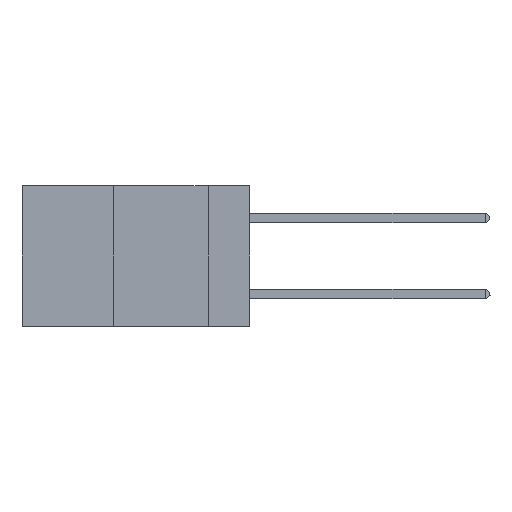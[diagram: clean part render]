
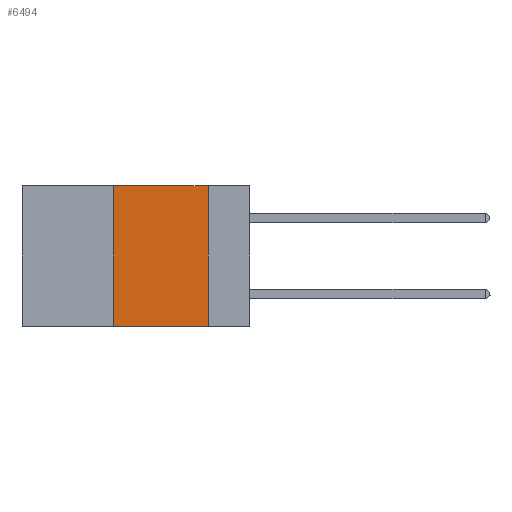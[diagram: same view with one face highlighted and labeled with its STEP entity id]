
A CAD part, left-side view. The second image highlights one B-rep face of the part: STEP entity #6494.
In plain terms, the highlighted planar face has unit normal (-1, 0, 0).
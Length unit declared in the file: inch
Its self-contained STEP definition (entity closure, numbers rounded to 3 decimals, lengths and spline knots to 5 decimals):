
#1934 = EDGE_CURVE ( 'NONE', #23274, #36076, #28534, .T. ) ;
#2976 = CARTESIAN_POINT ( 'NONE',  ( 0., 0.6, -0.37 ) ) ;
#3946 = EDGE_CURVE ( 'NONE', #43047, #36076, #5324, .T. ) ;
#4141 = VERTEX_POINT ( 'NONE', #40222 ) ;
#5134 = CARTESIAN_POINT ( 'NONE',  ( 0., 0.6, 0. ) ) ;
#5295 = DIRECTION ( 'NONE',  ( 1., 0., 0. ) ) ;
#5324 = LINE ( 'NONE', #2976, #43604 ) ;
#5707 = ORIENTED_EDGE ( 'NONE', *, *, #1934, .F. ) ;
#6494 = ADVANCED_FACE ( 'NONE', ( #9236 ), #23771, .F. ) ;
#8316 = EDGE_CURVE ( 'NONE', #43047, #4141, #22186, .T. ) ;
#9236 = FACE_OUTER_BOUND ( 'NONE', #27801, .T. ) ;
#12374 = VECTOR ( 'NONE', #16352, 39.37008 ) ;
#13719 = CARTESIAN_POINT ( 'NONE',  ( 0., 0.11, 0. ) ) ;
#15211 = ORIENTED_EDGE ( 'NONE', *, *, #3946, .T. ) ;
#15597 = DIRECTION ( 'NONE',  ( 0., -1., 0. ) ) ;
#16249 = CARTESIAN_POINT ( 'NONE',  ( 0., 0.11, 0. ) ) ;
#16352 = DIRECTION ( 'NONE',  ( 0., 0., 1. ) ) ;
#22186 = LINE ( 'NONE', #23783, #12374 ) ;
#23274 = VERTEX_POINT ( 'NONE', #16249 ) ;
#23771 = PLANE ( 'NONE',  #27609 ) ;
#23783 = CARTESIAN_POINT ( 'NONE',  ( 0., 0.36, 0. ) ) ;
#25252 = DIRECTION ( 'NONE',  ( 0., -1., 0. ) ) ;
#25569 = LINE ( 'NONE', #44047, #34938 ) ;
#27609 = AXIS2_PLACEMENT_3D ( 'NONE', #5134, #5295, #30923 ) ;
#27801 = EDGE_LOOP ( 'NONE', ( #5707, #35394, #39061, #15211 ) ) ;
#28534 = LINE ( 'NONE', #13719, #45943 ) ;
#28768 = CARTESIAN_POINT ( 'NONE',  ( 0., 0.11, -0.37 ) ) ;
#30923 = DIRECTION ( 'NONE',  ( 0., 0., -1. ) ) ;
#33296 = EDGE_CURVE ( 'NONE', #4141, #23274, #25569, .T. ) ;
#34938 = VECTOR ( 'NONE', #15597, 39.37008 ) ;
#35286 = DIRECTION ( 'NONE',  ( 0., 0., -1. ) ) ;
#35394 = ORIENTED_EDGE ( 'NONE', *, *, #33296, .F. ) ;
#36076 = VERTEX_POINT ( 'NONE', #28768 ) ;
#39061 = ORIENTED_EDGE ( 'NONE', *, *, #8316, .F. ) ;
#40222 = CARTESIAN_POINT ( 'NONE',  ( 0., 0.36, 0. ) ) ;
#41481 = CARTESIAN_POINT ( 'NONE',  ( 0., 0.36, -0.37 ) ) ;
#43047 = VERTEX_POINT ( 'NONE', #41481 ) ;
#43604 = VECTOR ( 'NONE', #25252, 39.37008 ) ;
#44047 = CARTESIAN_POINT ( 'NONE',  ( 0., 0.6, 0. ) ) ;
#45943 = VECTOR ( 'NONE', #35286, 39.37008 ) ;
